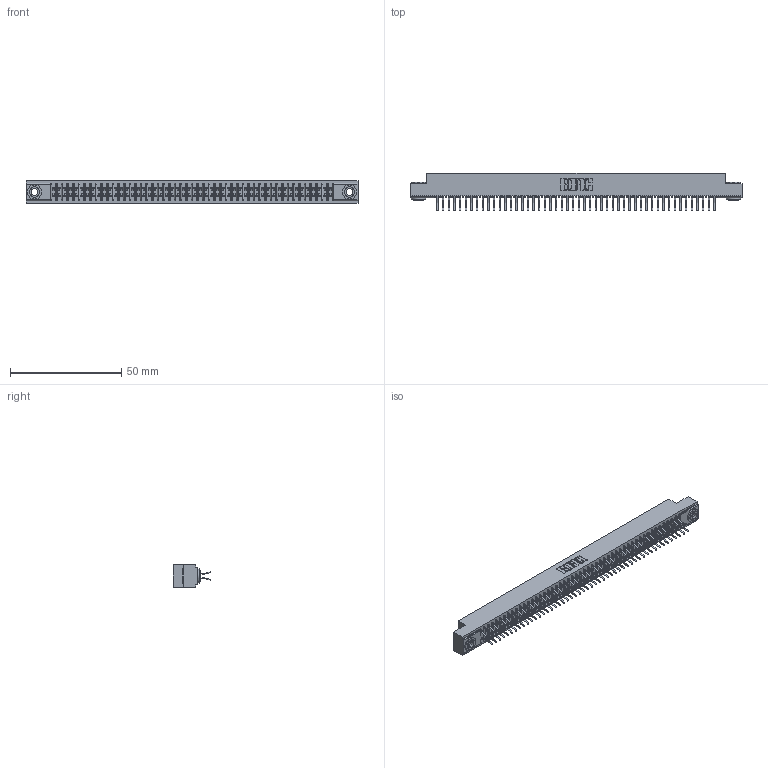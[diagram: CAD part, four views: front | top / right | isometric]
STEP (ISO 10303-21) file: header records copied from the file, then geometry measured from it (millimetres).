
FILE_DESCRIPTION (( 'STEP AP203' ), '1' );
FILE_NAME ('341-100-556-203.STEP', '2018-08-08T03:00:51', ( '' ), ( '' ), 'SwSTEP 2.0', 'SolidWorks 2016', '' );
FILE_SCHEMA (( 'CONFIG_CONTROL_DESIGN' ));
Length unit declared in the file: inch
Products named in the file (4): 345-250-002_345-250-002-102; 341-100-556-203; 341-292-001_341-292-156; 341 Part_.156 (3.96) Dia Mounting Holes
Assembly tree (103 placements, depth 2):
  341-100-556-203
    341 Part_.156 (3.96) Dia Mounting Holes
    341-292-001_341-292-156  x100
    345-250-002_345-250-002-102  x2
Bounding box: 149.22 x 17.07 x 10.16 mm (x, y, z)
Volume: 11059.7 mm3; surface area: 20368.3 mm2
Topology: 103 solids, 103 shells, 7168 faces, 20778 edges, 13478 vertices
Faces by surface type: plane 4092, cylinder 2868, sphere 102, torus 98, cone 8
Entity records: 60650 total; most frequent: CARTESIAN_POINT 10063, ORIENTED_EDGE 9992, DIRECTION 9780, EDGE_CURVE 4996, VECTOR 4030, LINE 4030, VERTEX_POINT 3158, AXIS2_PLACEMENT_3D 2875
